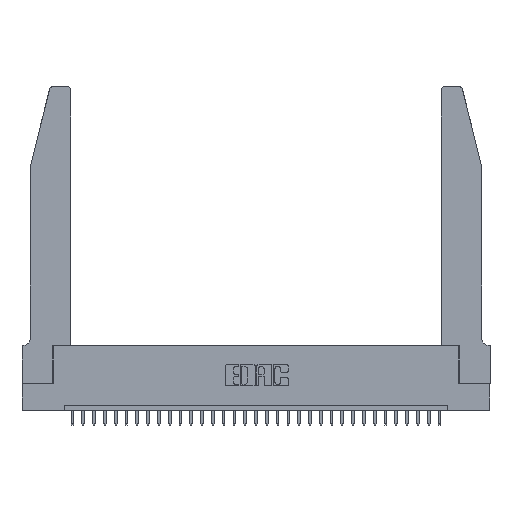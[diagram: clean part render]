
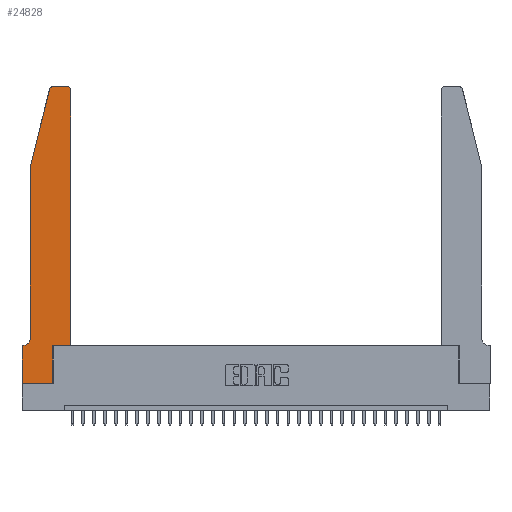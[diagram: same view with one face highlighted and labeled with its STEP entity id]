
A CAD part, top view. The second image highlights one B-rep face of the part: STEP entity #24828.
In plain terms, the highlighted planar face has unit normal (0, 0, 1).
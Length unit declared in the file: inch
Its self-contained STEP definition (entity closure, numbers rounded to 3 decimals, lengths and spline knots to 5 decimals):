
#425 = EDGE_CURVE ( 'NONE', #17786, #11817, #26415, .T. ) ;
#581 = ORIENTED_EDGE ( 'NONE', *, *, #425, .T. ) ;
#937 = CARTESIAN_POINT ( 'NONE',  ( 0., 0., 0.37 ) ) ;
#1563 = VERTEX_POINT ( 'NONE', #25088 ) ;
#1714 = DIRECTION ( 'NONE',  ( 0., 0., 1. ) ) ;
#1875 = LINE ( 'NONE', #10365, #9604 ) ;
#2131 = ORIENTED_EDGE ( 'NONE', *, *, #4224, .T. ) ;
#2338 = CARTESIAN_POINT ( 'NONE',  ( 0.0755, 2., 0.37 ) ) ;
#2681 = VECTOR ( 'NONE', #18369, 39.37008 ) ;
#2917 = EDGE_CURVE ( 'NONE', #18809, #10354, #1875, .T. ) ;
#3648 = DIRECTION ( 'NONE',  ( 0., 0., 1. ) ) ;
#3723 = ORIENTED_EDGE ( 'NONE', *, *, #5707, .T. ) ;
#3874 = EDGE_CURVE ( 'NONE', #20041, #17786, #22345, .T. ) ;
#3975 = CARTESIAN_POINT ( 'NONE',  ( 0., 0., 0.37 ) ) ;
#4002 = DIRECTION ( 'NONE',  ( -1., 0., 0. ) ) ;
#4076 = LINE ( 'NONE', #24705, #11412 ) ;
#4224 = EDGE_CURVE ( 'NONE', #1563, #23779, #23051, .T. ) ;
#4934 = VERTEX_POINT ( 'NONE', #29833 ) ;
#5457 = VERTEX_POINT ( 'NONE', #2338 ) ;
#5494 = VECTOR ( 'NONE', #21455, 39.37008 ) ;
#5571 = CARTESIAN_POINT ( 'NONE',  ( 0., 0.35, 0.37 ) ) ;
#5707 = EDGE_CURVE ( 'NONE', #11817, #5457, #4076, .T. ) ;
#6003 = ORIENTED_EDGE ( 'NONE', *, *, #2917, .T. ) ;
#6400 = CIRCLE ( 'NONE', #17529, 0.03 ) ;
#6639 = AXIS2_PLACEMENT_3D ( 'NONE', #18430, #3648, #16189 ) ;
#6954 = EDGE_CURVE ( 'NONE', #10354, #20041, #6400, .T. ) ;
#7567 = EDGE_CURVE ( 'NONE', #20229, #23319, #28047, .T. ) ;
#8105 = CARTESIAN_POINT ( 'NONE',  ( 0.4205, 2.75, 0.37 ) ) ;
#8401 = EDGE_CURVE ( 'NONE', #23319, #9798, #17147, .T. ) ;
#8575 = ORIENTED_EDGE ( 'NONE', *, *, #6954, .T. ) ;
#9303 = CARTESIAN_POINT ( 'NONE',  ( 0.0755, 2., 0.37 ) ) ;
#9604 = VECTOR ( 'NONE', #12868, 39.37008 ) ;
#9798 = VERTEX_POINT ( 'NONE', #22504 ) ;
#10354 = VERTEX_POINT ( 'NONE', #22780 ) ;
#10365 = CARTESIAN_POINT ( 'NONE',  ( 0.4505, 0.35, 0.37 ) ) ;
#10408 = ORIENTED_EDGE ( 'NONE', *, *, #3874, .T. ) ;
#10564 = VECTOR ( 'NONE', #30409, 39.37008 ) ;
#10907 = CARTESIAN_POINT ( 'NONE',  ( 0.284, 2.75, 0.37 ) ) ;
#11127 = VECTOR ( 'NONE', #14892, 39.37008 ) ;
#11343 = CARTESIAN_POINT ( 'NONE',  ( 0.0055, 0.42, 0.37 ) ) ;
#11412 = VECTOR ( 'NONE', #19941, 39.37008 ) ;
#11817 = VERTEX_POINT ( 'NONE', #21538 ) ;
#11909 = VECTOR ( 'NONE', #25282, 39.37008 ) ;
#12868 = DIRECTION ( 'NONE',  ( 0., 1., 0. ) ) ;
#14892 = DIRECTION ( 'NONE',  ( 1., 0., 0. ) ) ;
#15124 = ORIENTED_EDGE ( 'NONE', *, *, #20887, .T. ) ;
#16131 = CARTESIAN_POINT ( 'NONE',  ( 0.4505, 0.35, 0.37 ) ) ;
#16189 = DIRECTION ( 'NONE',  ( 1., 0., 0. ) ) ;
#16415 = DIRECTION ( 'NONE',  ( -1., 0., 0. ) ) ;
#17147 = LINE ( 'NONE', #30195, #10564 ) ;
#17500 = FACE_OUTER_BOUND ( 'NONE', #23264, .T. ) ;
#17529 = AXIS2_PLACEMENT_3D ( 'NONE', #31432, #1714, #23626 ) ;
#17581 = EDGE_CURVE ( 'NONE', #5457, #20229, #18438, .T. ) ;
#17786 = VERTEX_POINT ( 'NONE', #10907 ) ;
#18369 = DIRECTION ( 'NONE',  ( 1., 0., 0. ) ) ;
#18430 = CARTESIAN_POINT ( 'NONE',  ( 0.284, 2.72, 0.37 ) ) ;
#18438 = LINE ( 'NONE', #9303, #11909 ) ;
#18809 = VERTEX_POINT ( 'NONE', #21649 ) ;
#19091 = DIRECTION ( 'NONE',  ( 0., 1., 0. ) ) ;
#19123 = CARTESIAN_POINT ( 'NONE',  ( 0.2865, 0., 0.37 ) ) ;
#19941 = DIRECTION ( 'NONE',  ( -0.239, -0.971, 0. ) ) ;
#19988 = VECTOR ( 'NONE', #16415, 39.37008 ) ;
#20041 = VERTEX_POINT ( 'NONE', #8105 ) ;
#20155 = LINE ( 'NONE', #3975, #5494 ) ;
#20229 = VERTEX_POINT ( 'NONE', #26380 ) ;
#20547 = DIRECTION ( 'NONE',  ( 1., 0., 0. ) ) ;
#20870 = AXIS2_PLACEMENT_3D ( 'NONE', #5571, #27922, #20547 ) ;
#20887 = EDGE_CURVE ( 'NONE', #9798, #1563, #20155, .T. ) ;
#21455 = DIRECTION ( 'NONE',  ( 0., -1., 0. ) ) ;
#21538 = CARTESIAN_POINT ( 'NONE',  ( 0.25487, 2.72718, 0.37 ) ) ;
#21649 = CARTESIAN_POINT ( 'NONE',  ( 0.4505, 0.35, 0.37 ) ) ;
#22345 = LINE ( 'NONE', #25918, #19988 ) ;
#22504 = CARTESIAN_POINT ( 'NONE',  ( 0., 0.35, 0.37 ) ) ;
#22518 = EDGE_CURVE ( 'NONE', #4934, #18809, #25094, .T. ) ;
#22698 = AXIS2_PLACEMENT_3D ( 'NONE', #11343, #23720, #4002 ) ;
#22780 = CARTESIAN_POINT ( 'NONE',  ( 0.4505, 2.72, 0.37 ) ) ;
#23051 = LINE ( 'NONE', #937, #11127 ) ;
#23171 = VECTOR ( 'NONE', #19091, 39.37008 ) ;
#23264 = EDGE_LOOP ( 'NONE', ( #10408, #581, #3723, #27417, #27970, #29086, #15124, #2131, #26895, #24635, #6003, #8575 ) ) ;
#23319 = VERTEX_POINT ( 'NONE', #24447 ) ;
#23626 = DIRECTION ( 'NONE',  ( 1., 0., 0. ) ) ;
#23720 = DIRECTION ( 'NONE',  ( 0., 0., -1. ) ) ;
#23779 = VERTEX_POINT ( 'NONE', #19123 ) ;
#24447 = CARTESIAN_POINT ( 'NONE',  ( 0.0055, 0.35, 0.37 ) ) ;
#24635 = ORIENTED_EDGE ( 'NONE', *, *, #22518, .T. ) ;
#24705 = CARTESIAN_POINT ( 'NONE',  ( 0.0755, 2., 0.37 ) ) ;
#24828 = ADVANCED_FACE ( 'NONE', ( #17500 ), #30489, .T. ) ;
#25088 = CARTESIAN_POINT ( 'NONE',  ( 0., 0., 0.37 ) ) ;
#25094 = LINE ( 'NONE', #16131, #2681 ) ;
#25282 = DIRECTION ( 'NONE',  ( 0., -1., 0. ) ) ;
#25918 = CARTESIAN_POINT ( 'NONE',  ( 0.2605, 2.75, 0.37 ) ) ;
#26380 = CARTESIAN_POINT ( 'NONE',  ( 0.0755, 0.42, 0.37 ) ) ;
#26415 = CIRCLE ( 'NONE', #6639, 0.03 ) ;
#26895 = ORIENTED_EDGE ( 'NONE', *, *, #28551, .T. ) ;
#27417 = ORIENTED_EDGE ( 'NONE', *, *, #17581, .T. ) ;
#27922 = DIRECTION ( 'NONE',  ( 0., 0., 1. ) ) ;
#27970 = ORIENTED_EDGE ( 'NONE', *, *, #7567, .T. ) ;
#28047 = CIRCLE ( 'NONE', #22698, 0.07 ) ;
#28551 = EDGE_CURVE ( 'NONE', #23779, #4934, #29779, .T. ) ;
#28589 = CARTESIAN_POINT ( 'NONE',  ( 0.2865, 0.35, 0.37 ) ) ;
#29086 = ORIENTED_EDGE ( 'NONE', *, *, #8401, .T. ) ;
#29779 = LINE ( 'NONE', #28589, #23171 ) ;
#29833 = CARTESIAN_POINT ( 'NONE',  ( 0.2865, 0.35, 0.37 ) ) ;
#30195 = CARTESIAN_POINT ( 'NONE',  ( 0.0755, 0.35, 0.37 ) ) ;
#30409 = DIRECTION ( 'NONE',  ( -1., 0., 0. ) ) ;
#30489 = PLANE ( 'NONE',  #20870 ) ;
#31432 = CARTESIAN_POINT ( 'NONE',  ( 0.4205, 2.72, 0.37 ) ) ;
